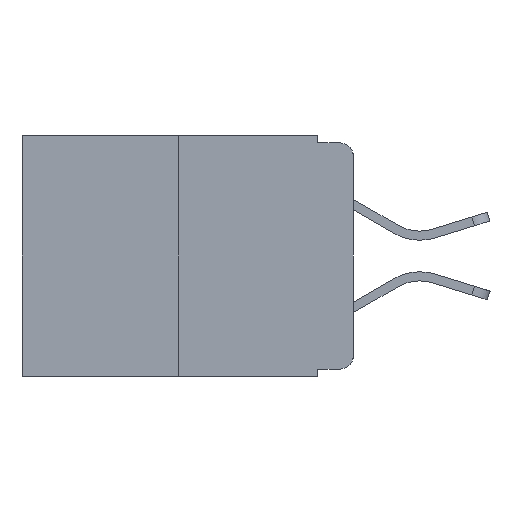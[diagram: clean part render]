
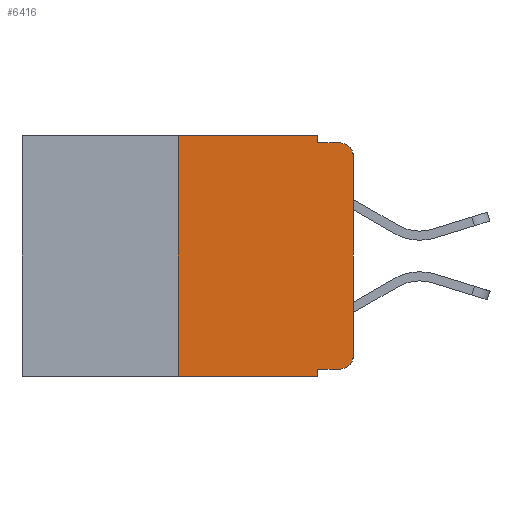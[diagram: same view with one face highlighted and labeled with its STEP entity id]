
A CAD part, left-side view. The second image highlights one B-rep face of the part: STEP entity #6416.
In plain terms, the highlighted planar face has unit normal (-1, 0, 0).
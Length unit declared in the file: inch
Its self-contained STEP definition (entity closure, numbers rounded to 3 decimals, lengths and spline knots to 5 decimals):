
#8 = DIRECTION ( 'NONE',  ( 0., 0., -1. ) ) ;
#102 = DIRECTION ( 'NONE',  ( 0., 0., 1. ) ) ;
#375 = VERTEX_POINT ( 'NONE', #6467 ) ;
#395 = VECTOR ( 'NONE', #6178, 39.37008 ) ;
#463 = LINE ( 'NONE', #2958, #9715 ) ;
#725 = CARTESIAN_POINT ( 'NONE',  ( 0., 0.473, -0.343 ) ) ;
#877 = ORIENTED_EDGE ( 'NONE', *, *, #2073, .T. ) ;
#996 = DIRECTION ( 'NONE',  ( 0., 0., 1. ) ) ;
#1090 = CARTESIAN_POINT ( 'NONE',  ( 0., 0.02, -0.333 ) ) ;
#1258 = ORIENTED_EDGE ( 'NONE', *, *, #10759, .T. ) ;
#1466 = VERTEX_POINT ( 'NONE', #4075 ) ;
#1795 = CARTESIAN_POINT ( 'NONE',  ( 0., 0.473, 0. ) ) ;
#1938 = VERTEX_POINT ( 'NONE', #4590 ) ;
#2073 = EDGE_CURVE ( 'NONE', #11056, #10339, #6483, .T. ) ;
#2212 = DIRECTION ( 'NONE',  ( 0., -1., 0. ) ) ;
#2254 = CARTESIAN_POINT ( 'NONE',  ( 0., 0.02, -0.03 ) ) ;
#2607 = VECTOR ( 'NONE', #3477, 39.37008 ) ;
#2634 = ORIENTED_EDGE ( 'NONE', *, *, #8955, .T. ) ;
#2883 = DIRECTION ( 'NONE',  ( 1., 0., 0. ) ) ;
#2958 = CARTESIAN_POINT ( 'NONE',  ( 0., 0., 0. ) ) ;
#3044 = CARTESIAN_POINT ( 'NONE',  ( 0., 0.25, 0. ) ) ;
#3457 = ORIENTED_EDGE ( 'NONE', *, *, #7109, .F. ) ;
#3477 = DIRECTION ( 'NONE',  ( 0., -1., 0. ) ) ;
#3533 = LINE ( 'NONE', #5632, #11808 ) ;
#3582 = LINE ( 'NONE', #5103, #395 ) ;
#3795 = CARTESIAN_POINT ( 'NONE',  ( 0., 0.02, -0.313 ) ) ;
#4057 = ORIENTED_EDGE ( 'NONE', *, *, #10879, .F. ) ;
#4075 = CARTESIAN_POINT ( 'NONE',  ( 0., 0.051, -0.343 ) ) ;
#4197 = LINE ( 'NONE', #7564, #5790 ) ;
#4571 = ORIENTED_EDGE ( 'NONE', *, *, #11099, .T. ) ;
#4590 = CARTESIAN_POINT ( 'NONE',  ( 0., 0.25, -0.343 ) ) ;
#4670 = VECTOR ( 'NONE', #12184, 39.37008 ) ;
#5000 = EDGE_CURVE ( 'NONE', #5964, #6274, #11883, .T. ) ;
#5076 = CIRCLE ( 'NONE', #6904, 0.02 ) ;
#5103 = CARTESIAN_POINT ( 'NONE',  ( 0., 0.051, 0. ) ) ;
#5609 = CARTESIAN_POINT ( 'NONE',  ( 0., 0.473, 0. ) ) ;
#5632 = CARTESIAN_POINT ( 'NONE',  ( 0., 0.051, 0. ) ) ;
#5695 = DIRECTION ( 'NONE',  ( 0., 0., -1. ) ) ;
#5790 = VECTOR ( 'NONE', #996, 39.37008 ) ;
#5964 = VERTEX_POINT ( 'NONE', #6080 ) ;
#5969 = VECTOR ( 'NONE', #2212, 39.37008 ) ;
#6036 = DIRECTION ( 'NONE',  ( -1., 0., 0. ) ) ;
#6080 = CARTESIAN_POINT ( 'NONE',  ( 0., 0.051, -0.01 ) ) ;
#6178 = DIRECTION ( 'NONE',  ( 0., 0., -1. ) ) ;
#6210 = AXIS2_PLACEMENT_3D ( 'NONE', #3795, #6685, #5695 ) ;
#6274 = VERTEX_POINT ( 'NONE', #9774 ) ;
#6414 = DIRECTION ( 'NONE',  ( 0., -1., 0. ) ) ;
#6416 = ADVANCED_FACE ( 'NONE', ( #10820 ), #11276, .F. ) ;
#6456 = LINE ( 'NONE', #1795, #4670 ) ;
#6467 = CARTESIAN_POINT ( 'NONE',  ( 0., 0.051, 0. ) ) ;
#6483 = CIRCLE ( 'NONE', #6210, 0.02 ) ;
#6685 = DIRECTION ( 'NONE',  ( -1., 0., 0. ) ) ;
#6904 = AXIS2_PLACEMENT_3D ( 'NONE', #2254, #6036, #7987 ) ;
#7109 = EDGE_CURVE ( 'NONE', #10113, #1466, #3533, .T. ) ;
#7168 = ORIENTED_EDGE ( 'NONE', *, *, #10613, .F. ) ;
#7348 = CARTESIAN_POINT ( 'NONE',  ( 0., 0., -0.03 ) ) ;
#7408 = CARTESIAN_POINT ( 'NONE',  ( 0., 0.051, -0.333 ) ) ;
#7523 = VERTEX_POINT ( 'NONE', #7348 ) ;
#7564 = CARTESIAN_POINT ( 'NONE',  ( 0., 0.25, 0. ) ) ;
#7987 = DIRECTION ( 'NONE',  ( 0., 0., -1. ) ) ;
#8220 = VERTEX_POINT ( 'NONE', #3044 ) ;
#8257 = ORIENTED_EDGE ( 'NONE', *, *, #8372, .F. ) ;
#8372 = EDGE_CURVE ( 'NONE', #8220, #375, #6456, .T. ) ;
#8373 = DIRECTION ( 'NONE',  ( 0., 0., -1. ) ) ;
#8470 = EDGE_LOOP ( 'NONE', ( #10545, #4571, #11552, #7168, #8257, #4057, #1258, #3457, #2634, #877 ) ) ;
#8657 = EDGE_CURVE ( 'NONE', #10339, #7523, #463, .T. ) ;
#8955 = EDGE_CURVE ( 'NONE', #10113, #11056, #9243, .T. ) ;
#9243 = LINE ( 'NONE', #7408, #2607 ) ;
#9654 = VECTOR ( 'NONE', #6414, 39.37008 ) ;
#9715 = VECTOR ( 'NONE', #102, 39.37008 ) ;
#9734 = CARTESIAN_POINT ( 'NONE',  ( 0., 0.051, -0.01 ) ) ;
#9774 = CARTESIAN_POINT ( 'NONE',  ( 0., 0.02, -0.01 ) ) ;
#10113 = VERTEX_POINT ( 'NONE', #10118 ) ;
#10118 = CARTESIAN_POINT ( 'NONE',  ( 0., 0.051, -0.333 ) ) ;
#10339 = VERTEX_POINT ( 'NONE', #11340 ) ;
#10545 = ORIENTED_EDGE ( 'NONE', *, *, #8657, .T. ) ;
#10613 = EDGE_CURVE ( 'NONE', #375, #5964, #3582, .T. ) ;
#10734 = AXIS2_PLACEMENT_3D ( 'NONE', #5609, #2883, #8373 ) ;
#10759 = EDGE_CURVE ( 'NONE', #1938, #1466, #11735, .T. ) ;
#10820 = FACE_OUTER_BOUND ( 'NONE', #8470, .T. ) ;
#10879 = EDGE_CURVE ( 'NONE', #1938, #8220, #4197, .T. ) ;
#11056 = VERTEX_POINT ( 'NONE', #1090 ) ;
#11099 = EDGE_CURVE ( 'NONE', #7523, #6274, #5076, .T. ) ;
#11276 = PLANE ( 'NONE',  #10734 ) ;
#11340 = CARTESIAN_POINT ( 'NONE',  ( 0., 0., -0.313 ) ) ;
#11552 = ORIENTED_EDGE ( 'NONE', *, *, #5000, .F. ) ;
#11735 = LINE ( 'NONE', #725, #9654 ) ;
#11808 = VECTOR ( 'NONE', #8, 39.37008 ) ;
#11883 = LINE ( 'NONE', #9734, #5969 ) ;
#12184 = DIRECTION ( 'NONE',  ( 0., -1., 0. ) ) ;
